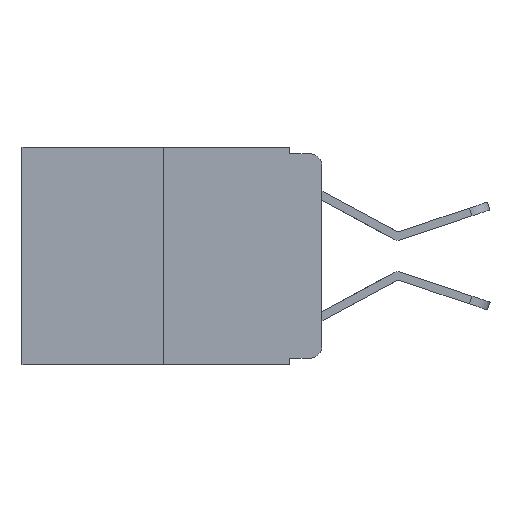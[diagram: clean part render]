
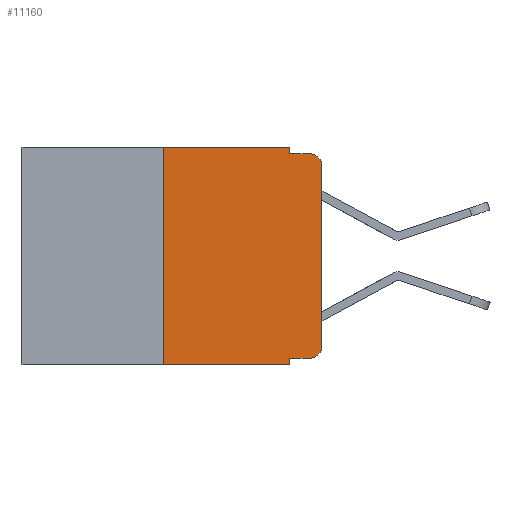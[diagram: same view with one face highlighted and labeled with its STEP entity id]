
A CAD part, left-side view. The second image highlights one B-rep face of the part: STEP entity #11160.
In plain terms, the highlighted planar face has unit normal (-1, 0, 0).
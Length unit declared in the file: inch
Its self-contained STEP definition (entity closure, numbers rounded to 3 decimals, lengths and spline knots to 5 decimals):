
#28 = PLANE ( 'NONE',  #70 ) ;
#65 = CARTESIAN_POINT ( 'NONE',  ( 0., 0.25, 0. ) ) ;
#70 = AXIS2_PLACEMENT_3D ( 'NONE', #1154, #8403, #2238 ) ;
#150 = CARTESIAN_POINT ( 'NONE',  ( 0., 0.25, 0. ) ) ;
#299 = DIRECTION ( 'NONE',  ( 0., 0., 1. ) ) ;
#530 = VECTOR ( 'NONE', #299, 39.37008 ) ;
#607 = LINE ( 'NONE', #2659, #3037 ) ;
#722 = VECTOR ( 'NONE', #5704, 39.37008 ) ;
#790 = ORIENTED_EDGE ( 'NONE', *, *, #12837, .T. ) ;
#911 = VERTEX_POINT ( 'NONE', #1570 ) ;
#1088 = ORIENTED_EDGE ( 'NONE', *, *, #9546, .F. ) ;
#1154 = CARTESIAN_POINT ( 'NONE',  ( 0., 0.473, 0. ) ) ;
#1380 = DIRECTION ( 'NONE',  ( 0., -1., 0. ) ) ;
#1527 = DIRECTION ( 'NONE',  ( -1., 0., 0. ) ) ;
#1570 = CARTESIAN_POINT ( 'NONE',  ( 0., 0., -0.03 ) ) ;
#1705 = VECTOR ( 'NONE', #1380, 39.37008 ) ;
#1730 = CIRCLE ( 'NONE', #8073, 0.02 ) ;
#1898 = VERTEX_POINT ( 'NONE', #150 ) ;
#2047 = VECTOR ( 'NONE', #13347, 39.37008 ) ;
#2076 = CARTESIAN_POINT ( 'NONE',  ( 0., 0.02, -0.01 ) ) ;
#2238 = DIRECTION ( 'NONE',  ( 0., 0., -1. ) ) ;
#2339 = CARTESIAN_POINT ( 'NONE',  ( 0., 0., 0. ) ) ;
#2619 = CIRCLE ( 'NONE', #11582, 0.02 ) ;
#2659 = CARTESIAN_POINT ( 'NONE',  ( 0., 0.473, -0.343 ) ) ;
#2790 = LINE ( 'NONE', #2339, #530 ) ;
#2902 = CARTESIAN_POINT ( 'NONE',  ( 0., 0., -0.313 ) ) ;
#2924 = DIRECTION ( 'NONE',  ( -1., 0., 0. ) ) ;
#3037 = VECTOR ( 'NONE', #9910, 39.37008 ) ;
#3061 = VERTEX_POINT ( 'NONE', #7904 ) ;
#3062 = VECTOR ( 'NONE', #5640, 39.37008 ) ;
#3169 = EDGE_CURVE ( 'NONE', #911, #5855, #1730, .T. ) ;
#3171 = ORIENTED_EDGE ( 'NONE', *, *, #4586, .F. ) ;
#3959 = CARTESIAN_POINT ( 'NONE',  ( 0., 0.051, 0. ) ) ;
#4164 = EDGE_CURVE ( 'NONE', #5975, #5855, #6562, .T. ) ;
#4393 = CARTESIAN_POINT ( 'NONE',  ( 0., 0.02, -0.333 ) ) ;
#4492 = EDGE_CURVE ( 'NONE', #8865, #5975, #5258, .T. ) ;
#4586 = EDGE_CURVE ( 'NONE', #3061, #1898, #5099, .T. ) ;
#4903 = DIRECTION ( 'NONE',  ( 0., 0., -1. ) ) ;
#5099 = LINE ( 'NONE', #65, #2047 ) ;
#5258 = LINE ( 'NONE', #3959, #5770 ) ;
#5579 = CARTESIAN_POINT ( 'NONE',  ( 0., 0.051, -0.01 ) ) ;
#5640 = DIRECTION ( 'NONE',  ( 0., 0., -1. ) ) ;
#5647 = EDGE_CURVE ( 'NONE', #1898, #8865, #8982, .T. ) ;
#5704 = DIRECTION ( 'NONE',  ( 0., -1., 0. ) ) ;
#5770 = VECTOR ( 'NONE', #4903, 39.37008 ) ;
#5806 = CARTESIAN_POINT ( 'NONE',  ( 0., 0.473, 0. ) ) ;
#5849 = CARTESIAN_POINT ( 'NONE',  ( 0., 0.051, -0.333 ) ) ;
#5855 = VERTEX_POINT ( 'NONE', #2076 ) ;
#5876 = DIRECTION ( 'NONE',  ( 0., 0., -1. ) ) ;
#5975 = VERTEX_POINT ( 'NONE', #10697 ) ;
#6045 = CARTESIAN_POINT ( 'NONE',  ( 0., 0.051, 0. ) ) ;
#6311 = LINE ( 'NONE', #5849, #9396 ) ;
#6562 = LINE ( 'NONE', #5579, #1705 ) ;
#7188 = CARTESIAN_POINT ( 'NONE',  ( 0., 0.051, -0.343 ) ) ;
#7551 = EDGE_CURVE ( 'NONE', #9571, #911, #2790, .T. ) ;
#7740 = CARTESIAN_POINT ( 'NONE',  ( 0., 0.02, -0.313 ) ) ;
#7904 = CARTESIAN_POINT ( 'NONE',  ( 0., 0.25, -0.343 ) ) ;
#7998 = ORIENTED_EDGE ( 'NONE', *, *, #4492, .F. ) ;
#8073 = AXIS2_PLACEMENT_3D ( 'NONE', #12157, #2924, #12244 ) ;
#8359 = ORIENTED_EDGE ( 'NONE', *, *, #9214, .T. ) ;
#8403 = DIRECTION ( 'NONE',  ( 1., 0., 0. ) ) ;
#8580 = ORIENTED_EDGE ( 'NONE', *, *, #3169, .T. ) ;
#8687 = CARTESIAN_POINT ( 'NONE',  ( 0., 0.051, 0. ) ) ;
#8865 = VERTEX_POINT ( 'NONE', #6045 ) ;
#8982 = LINE ( 'NONE', #5806, #722 ) ;
#9105 = VERTEX_POINT ( 'NONE', #4393 ) ;
#9214 = EDGE_CURVE ( 'NONE', #10450, #9105, #6311, .T. ) ;
#9396 = VECTOR ( 'NONE', #10850, 39.37008 ) ;
#9546 = EDGE_CURVE ( 'NONE', #10450, #11061, #12724, .T. ) ;
#9571 = VERTEX_POINT ( 'NONE', #2902 ) ;
#9910 = DIRECTION ( 'NONE',  ( 0., -1., 0. ) ) ;
#10101 = CARTESIAN_POINT ( 'NONE',  ( 0., 0.051, -0.333 ) ) ;
#10104 = EDGE_CURVE ( 'NONE', #3061, #11061, #607, .T. ) ;
#10450 = VERTEX_POINT ( 'NONE', #10101 ) ;
#10506 = ORIENTED_EDGE ( 'NONE', *, *, #10104, .T. ) ;
#10697 = CARTESIAN_POINT ( 'NONE',  ( 0., 0.051, -0.01 ) ) ;
#10850 = DIRECTION ( 'NONE',  ( 0., -1., 0. ) ) ;
#10928 = ORIENTED_EDGE ( 'NONE', *, *, #5647, .F. ) ;
#11061 = VERTEX_POINT ( 'NONE', #7188 ) ;
#11160 = ADVANCED_FACE ( 'NONE', ( #11558 ), #28, .F. ) ;
#11558 = FACE_OUTER_BOUND ( 'NONE', #12784, .T. ) ;
#11582 = AXIS2_PLACEMENT_3D ( 'NONE', #7740, #1527, #5876 ) ;
#12157 = CARTESIAN_POINT ( 'NONE',  ( 0., 0.02, -0.03 ) ) ;
#12244 = DIRECTION ( 'NONE',  ( 0., 0., -1. ) ) ;
#12724 = LINE ( 'NONE', #8687, #3062 ) ;
#12784 = EDGE_LOOP ( 'NONE', ( #12849, #8580, #12985, #7998, #10928, #3171, #10506, #1088, #8359, #790 ) ) ;
#12837 = EDGE_CURVE ( 'NONE', #9105, #9571, #2619, .T. ) ;
#12849 = ORIENTED_EDGE ( 'NONE', *, *, #7551, .T. ) ;
#12985 = ORIENTED_EDGE ( 'NONE', *, *, #4164, .F. ) ;
#13347 = DIRECTION ( 'NONE',  ( 0., 0., 1. ) ) ;
